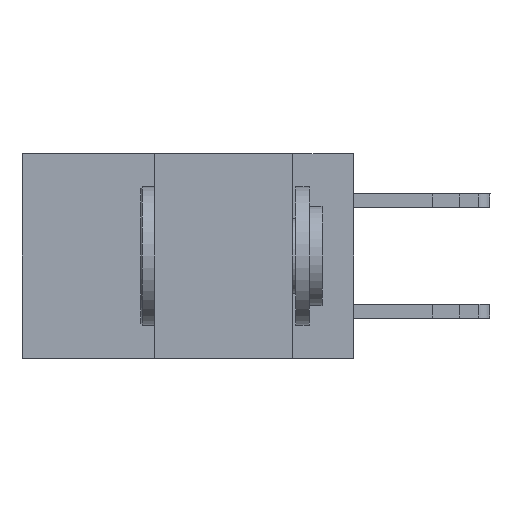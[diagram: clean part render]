
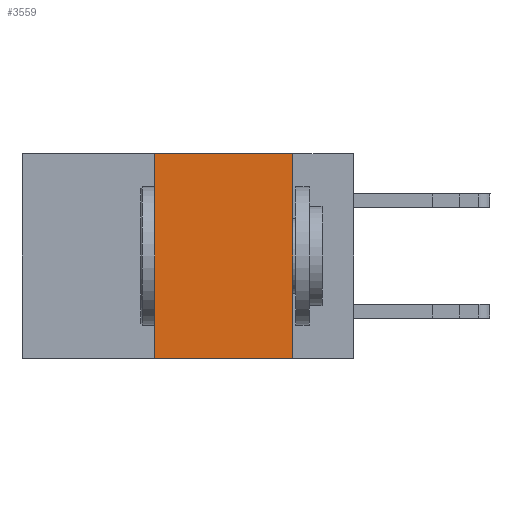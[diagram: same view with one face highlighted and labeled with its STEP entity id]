
A CAD part, left-side view. The second image highlights one B-rep face of the part: STEP entity #3559.
In plain terms, the highlighted planar face has unit normal (-1, 0, 0).
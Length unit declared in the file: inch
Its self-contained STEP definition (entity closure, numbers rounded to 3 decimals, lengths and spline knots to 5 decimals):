
#81 = CARTESIAN_POINT ( 'NONE',  ( 0., 0.11, 0. ) ) ;
#645 = ORIENTED_EDGE ( 'NONE', *, *, #21014, .T. ) ;
#1996 = EDGE_CURVE ( 'NONE', #28260, #13113, #13816, .T. ) ;
#3559 = ADVANCED_FACE ( 'NONE', ( #21085 ), #6988, .F. ) ;
#3796 = CARTESIAN_POINT ( 'NONE',  ( 0., 0.36, 0. ) ) ;
#4056 = VERTEX_POINT ( 'NONE', #27195 ) ;
#4852 = VECTOR ( 'NONE', #19002, 39.37008 ) ;
#6988 = PLANE ( 'NONE',  #28703 ) ;
#7077 = VERTEX_POINT ( 'NONE', #3796 ) ;
#7819 = CARTESIAN_POINT ( 'NONE',  ( 0., 0.36, 0. ) ) ;
#9393 = DIRECTION ( 'NONE',  ( 0., 0., -1. ) ) ;
#9608 = CARTESIAN_POINT ( 'NONE',  ( 0., 0.6, 0. ) ) ;
#9628 = CARTESIAN_POINT ( 'NONE',  ( 0., 0.11, -0.37 ) ) ;
#10081 = VECTOR ( 'NONE', #18831, 39.37008 ) ;
#11957 = DIRECTION ( 'NONE',  ( 0., 0., 1. ) ) ;
#12538 = CARTESIAN_POINT ( 'NONE',  ( 0., 0.6, -0.37 ) ) ;
#13113 = VERTEX_POINT ( 'NONE', #9628 ) ;
#13816 = LINE ( 'NONE', #27741, #23647 ) ;
#13833 = VECTOR ( 'NONE', #11957, 39.37008 ) ;
#15727 = ORIENTED_EDGE ( 'NONE', *, *, #22750, .F. ) ;
#18471 = ORIENTED_EDGE ( 'NONE', *, *, #1996, .F. ) ;
#18831 = DIRECTION ( 'NONE',  ( 0., -1., 0. ) ) ;
#19002 = DIRECTION ( 'NONE',  ( 0., -1., 0. ) ) ;
#19063 = DIRECTION ( 'NONE',  ( 0., 0., -1. ) ) ;
#19622 = EDGE_LOOP ( 'NONE', ( #18471, #15727, #28885, #645 ) ) ;
#21014 = EDGE_CURVE ( 'NONE', #4056, #13113, #25961, .T. ) ;
#21085 = FACE_OUTER_BOUND ( 'NONE', #19622, .T. ) ;
#22352 = LINE ( 'NONE', #9608, #10081 ) ;
#22750 = EDGE_CURVE ( 'NONE', #7077, #28260, #22352, .T. ) ;
#23647 = VECTOR ( 'NONE', #19063, 39.37008 ) ;
#24243 = EDGE_CURVE ( 'NONE', #4056, #7077, #26477, .T. ) ;
#25297 = CARTESIAN_POINT ( 'NONE',  ( 0., 0.6, 0. ) ) ;
#25961 = LINE ( 'NONE', #12538, #4852 ) ;
#26477 = LINE ( 'NONE', #7819, #13833 ) ;
#27195 = CARTESIAN_POINT ( 'NONE',  ( 0., 0.36, -0.37 ) ) ;
#27272 = DIRECTION ( 'NONE',  ( 1., 0., 0. ) ) ;
#27741 = CARTESIAN_POINT ( 'NONE',  ( 0., 0.11, 0. ) ) ;
#28260 = VERTEX_POINT ( 'NONE', #81 ) ;
#28703 = AXIS2_PLACEMENT_3D ( 'NONE', #25297, #27272, #9393 ) ;
#28885 = ORIENTED_EDGE ( 'NONE', *, *, #24243, .F. ) ;
